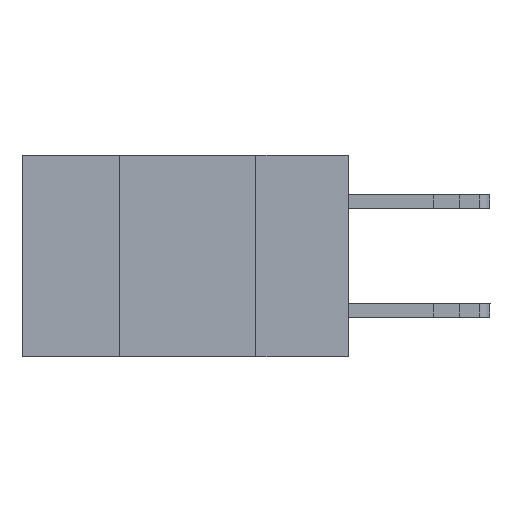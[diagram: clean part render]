
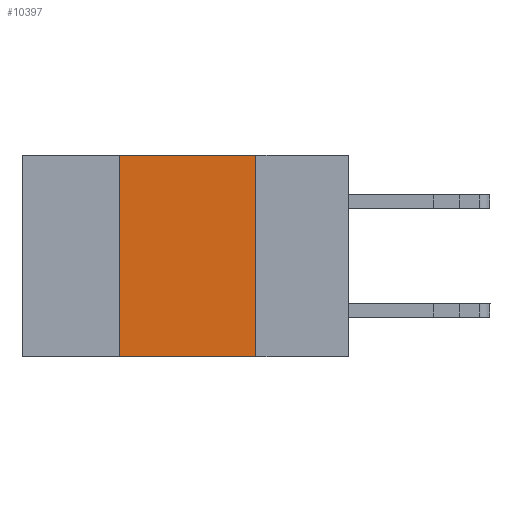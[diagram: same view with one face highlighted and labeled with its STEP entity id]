
A CAD part, left-side view. The second image highlights one B-rep face of the part: STEP entity #10397.
In plain terms, the highlighted planar face has unit normal (-1, 0, 0).
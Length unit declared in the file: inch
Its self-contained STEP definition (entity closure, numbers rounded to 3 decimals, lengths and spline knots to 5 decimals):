
#202 = VERTEX_POINT ( 'NONE', #6094 ) ;
#334 = PLANE ( 'NONE',  #11133 ) ;
#403 = DIRECTION ( 'NONE',  ( 0., 0., -1. ) ) ;
#536 = DIRECTION ( 'NONE',  ( 0., 0., 1. ) ) ;
#695 = ORIENTED_EDGE ( 'NONE', *, *, #998, .F. ) ;
#699 = ORIENTED_EDGE ( 'NONE', *, *, #4688, .F. ) ;
#732 = ORIENTED_EDGE ( 'NONE', *, *, #6469, .F. ) ;
#746 = ORIENTED_EDGE ( 'NONE', *, *, #7671, .T. ) ;
#998 = EDGE_CURVE ( 'NONE', #10260, #11819, #5438, .T. ) ;
#1388 = DIRECTION ( 'NONE',  ( 0., 0., -1. ) ) ;
#1814 = VECTOR ( 'NONE', #536, 39.37008 ) ;
#2584 = VERTEX_POINT ( 'NONE', #6757 ) ;
#3246 = CARTESIAN_POINT ( 'NONE',  ( 0., 0.6, 0. ) ) ;
#3292 = CARTESIAN_POINT ( 'NONE',  ( 0., 0.6, -0.37 ) ) ;
#3320 = CARTESIAN_POINT ( 'NONE',  ( 0., 0.6, 0. ) ) ;
#4323 = VECTOR ( 'NONE', #10506, 39.37008 ) ;
#4362 = CARTESIAN_POINT ( 'NONE',  ( 0., 0.17, -0.37 ) ) ;
#4613 = LINE ( 'NONE', #3320, #4323 ) ;
#4682 = FACE_OUTER_BOUND ( 'NONE', #4824, .T. ) ;
#4688 = EDGE_CURVE ( 'NONE', #202, #10260, #4613, .T. ) ;
#4824 = EDGE_LOOP ( 'NONE', ( #695, #699, #732, #746 ) ) ;
#5374 = VECTOR ( 'NONE', #6885, 39.37008 ) ;
#5438 = LINE ( 'NONE', #7521, #10206 ) ;
#6094 = CARTESIAN_POINT ( 'NONE',  ( 0., 0.42, 0. ) ) ;
#6469 = EDGE_CURVE ( 'NONE', #2584, #202, #11370, .T. ) ;
#6648 = CARTESIAN_POINT ( 'NONE',  ( 0., 0.17, 0. ) ) ;
#6757 = CARTESIAN_POINT ( 'NONE',  ( 0., 0.42, -0.37 ) ) ;
#6838 = DIRECTION ( 'NONE',  ( 1., 0., 0. ) ) ;
#6885 = DIRECTION ( 'NONE',  ( 0., -1., 0. ) ) ;
#7521 = CARTESIAN_POINT ( 'NONE',  ( 0., 0.17, -0.37 ) ) ;
#7671 = EDGE_CURVE ( 'NONE', #2584, #11819, #7738, .T. ) ;
#7738 = LINE ( 'NONE', #3292, #5374 ) ;
#10206 = VECTOR ( 'NONE', #403, 39.37008 ) ;
#10260 = VERTEX_POINT ( 'NONE', #6648 ) ;
#10397 = ADVANCED_FACE ( 'NONE', ( #4682 ), #334, .F. ) ;
#10506 = DIRECTION ( 'NONE',  ( 0., -1., 0. ) ) ;
#11133 = AXIS2_PLACEMENT_3D ( 'NONE', #3246, #6838, #1388 ) ;
#11370 = LINE ( 'NONE', #11424, #1814 ) ;
#11424 = CARTESIAN_POINT ( 'NONE',  ( 0., 0.42, -0.37 ) ) ;
#11819 = VERTEX_POINT ( 'NONE', #4362 ) ;
